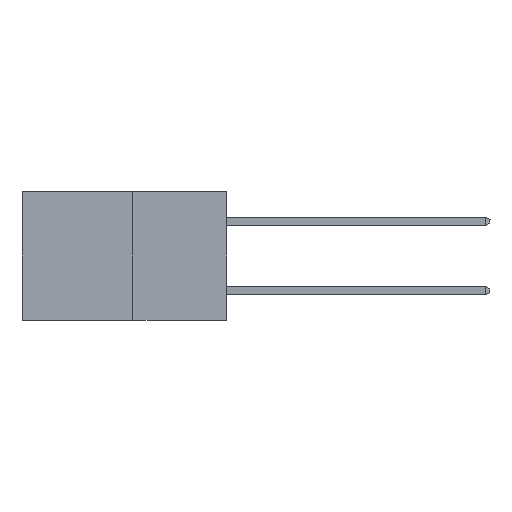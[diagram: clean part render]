
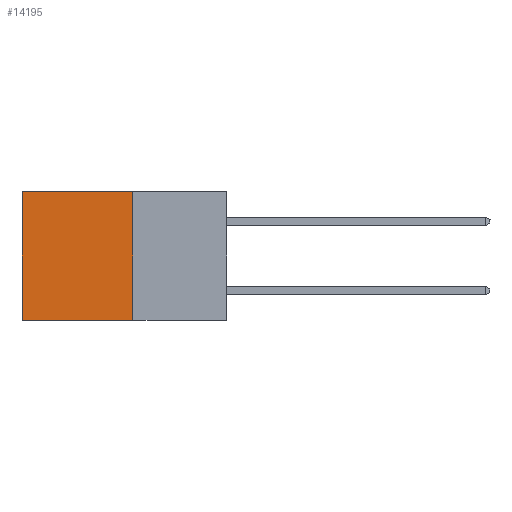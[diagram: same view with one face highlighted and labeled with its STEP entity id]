
A CAD part, left-side view. The second image highlights one B-rep face of the part: STEP entity #14195.
In plain terms, the highlighted planar face has unit normal (-1, 0, 0).
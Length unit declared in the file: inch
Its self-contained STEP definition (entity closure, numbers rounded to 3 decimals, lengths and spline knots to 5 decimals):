
#101 = CARTESIAN_POINT ( 'NONE',  ( 0.277, 0.27, -0.37 ) ) ;
#867 = LINE ( 'NONE', #101, #1383 ) ;
#951 = VERTEX_POINT ( 'NONE', #20729 ) ;
#1187 = EDGE_CURVE ( 'NONE', #8678, #14610, #13325, .T. ) ;
#1197 = EDGE_CURVE ( 'NONE', #8678, #951, #867, .T. ) ;
#1320 = ORIENTED_EDGE ( 'NONE', *, *, #1197, .F. ) ;
#1383 = VECTOR ( 'NONE', #2688, 39.37008 ) ;
#2125 = LINE ( 'NONE', #14210, #14561 ) ;
#2599 = PLANE ( 'NONE',  #18921 ) ;
#2688 = DIRECTION ( 'NONE',  ( 0., 0., -1. ) ) ;
#2760 = DIRECTION ( 'NONE',  ( 0., 1., 0. ) ) ;
#3315 = CARTESIAN_POINT ( 'NONE',  ( 0.277, 0.27, -0.37 ) ) ;
#4075 = ORIENTED_EDGE ( 'NONE', *, *, #17600, .T. ) ;
#4717 = EDGE_LOOP ( 'NONE', ( #4075, #19447, #1320, #7725 ) ) ;
#4970 = DIRECTION ( 'NONE',  ( 0., 1., 0. ) ) ;
#7593 = CARTESIAN_POINT ( 'NONE',  ( 0.277, 0.27, -0.37 ) ) ;
#7725 = ORIENTED_EDGE ( 'NONE', *, *, #1187, .T. ) ;
#8678 = VERTEX_POINT ( 'NONE', #15368 ) ;
#9121 = VECTOR ( 'NONE', #2760, 39.37008 ) ;
#9227 = DIRECTION ( 'NONE',  ( 0., 0., -1. ) ) ;
#10163 = VECTOR ( 'NONE', #4970, 39.37008 ) ;
#10645 = LINE ( 'NONE', #3315, #10163 ) ;
#12464 = VERTEX_POINT ( 'NONE', #16294 ) ;
#13237 = FACE_OUTER_BOUND ( 'NONE', #4717, .T. ) ;
#13325 = LINE ( 'NONE', #13866, #9121 ) ;
#13866 = CARTESIAN_POINT ( 'NONE',  ( 0.277, 0.27, 0. ) ) ;
#14195 = ADVANCED_FACE ( 'NONE', ( #13237 ), #2599, .F. ) ;
#14210 = CARTESIAN_POINT ( 'NONE',  ( 0.277, 0.59, -0.37 ) ) ;
#14561 = VECTOR ( 'NONE', #20622, 39.37008 ) ;
#14610 = VERTEX_POINT ( 'NONE', #16425 ) ;
#15368 = CARTESIAN_POINT ( 'NONE',  ( 0.277, 0.27, 0. ) ) ;
#16294 = CARTESIAN_POINT ( 'NONE',  ( 0.277, 0.59, -0.37 ) ) ;
#16354 = EDGE_CURVE ( 'NONE', #951, #12464, #10645, .T. ) ;
#16425 = CARTESIAN_POINT ( 'NONE',  ( 0.277, 0.59, 0. ) ) ;
#17600 = EDGE_CURVE ( 'NONE', #14610, #12464, #2125, .T. ) ;
#18766 = DIRECTION ( 'NONE',  ( 1., 0., 0. ) ) ;
#18921 = AXIS2_PLACEMENT_3D ( 'NONE', #7593, #18766, #9227 ) ;
#19447 = ORIENTED_EDGE ( 'NONE', *, *, #16354, .F. ) ;
#20622 = DIRECTION ( 'NONE',  ( 0., 0., -1. ) ) ;
#20729 = CARTESIAN_POINT ( 'NONE',  ( 0.277, 0.27, -0.37 ) ) ;
